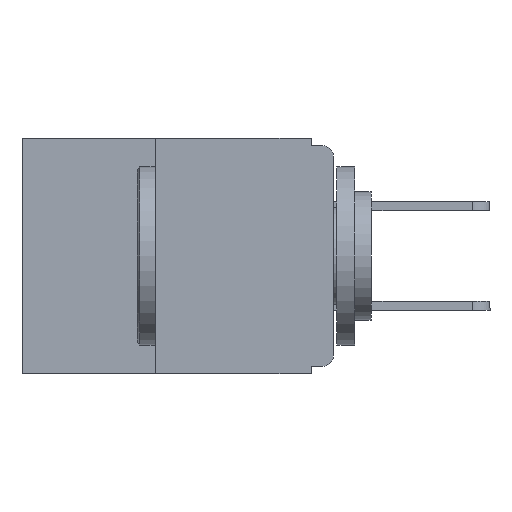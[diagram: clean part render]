
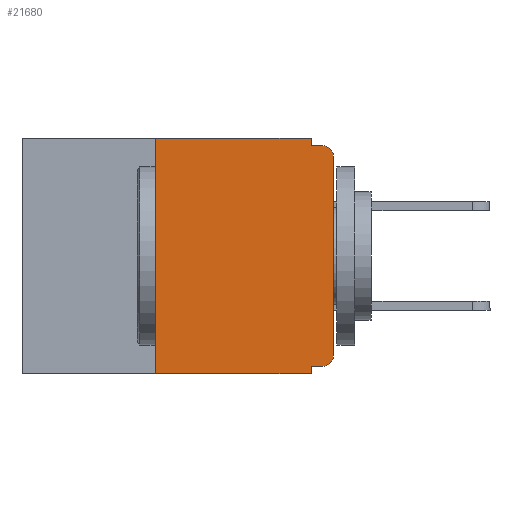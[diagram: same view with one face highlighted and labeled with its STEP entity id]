
A CAD part, left-side view. The second image highlights one B-rep face of the part: STEP entity #21680.
In plain terms, the highlighted planar face has unit normal (-1, 0, 0).
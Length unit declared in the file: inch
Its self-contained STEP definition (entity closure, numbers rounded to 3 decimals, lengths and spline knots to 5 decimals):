
#209 = PLANE ( 'NONE',  #31440 ) ;
#312 = DIRECTION ( 'NONE',  ( 0., 0., -1. ) ) ;
#1443 = AXIS2_PLACEMENT_3D ( 'NONE', #21757, #6638, #24270 ) ;
#2248 = ORIENTED_EDGE ( 'NONE', *, *, #5438, .T. ) ;
#3020 = VERTEX_POINT ( 'NONE', #16339 ) ;
#4085 = VECTOR ( 'NONE', #5358, 39.37008 ) ;
#4108 = DIRECTION ( 'NONE',  ( 0., 0., -1. ) ) ;
#4251 = ORIENTED_EDGE ( 'NONE', *, *, #12909, .F. ) ;
#4727 = CARTESIAN_POINT ( 'NONE',  ( 0., 0.437, -0.33 ) ) ;
#5188 = VECTOR ( 'NONE', #17422, 39.37008 ) ;
#5358 = DIRECTION ( 'NONE',  ( 0., 0., 1. ) ) ;
#5438 = EDGE_CURVE ( 'NONE', #30151, #17853, #26292, .T. ) ;
#6176 = DIRECTION ( 'NONE',  ( 0., 0., -1. ) ) ;
#6638 = DIRECTION ( 'NONE',  ( -1., 0., 0. ) ) ;
#7241 = VECTOR ( 'NONE', #6176, 39.37008 ) ;
#7500 = EDGE_CURVE ( 'NONE', #26751, #17238, #28093, .T. ) ;
#7616 = ORIENTED_EDGE ( 'NONE', *, *, #7500, .F. ) ;
#7727 = ORIENTED_EDGE ( 'NONE', *, *, #22279, .T. ) ;
#7857 = VERTEX_POINT ( 'NONE', #17319 ) ;
#8294 = ORIENTED_EDGE ( 'NONE', *, *, #17800, .F. ) ;
#9288 = VECTOR ( 'NONE', #27717, 39.37008 ) ;
#10606 = ORIENTED_EDGE ( 'NONE', *, *, #11639, .T. ) ;
#10917 = EDGE_LOOP ( 'NONE', ( #7727, #2248, #12436, #4251, #28418, #7616, #10606, #8294, #29253, #27120 ) ) ;
#10956 = EDGE_CURVE ( 'NONE', #32414, #18442, #30687, .T. ) ;
#11639 = EDGE_CURVE ( 'NONE', #26751, #3020, #24506, .T. ) ;
#12216 = EDGE_CURVE ( 'NONE', #32414, #7857, #21367, .T. ) ;
#12436 = ORIENTED_EDGE ( 'NONE', *, *, #16873, .F. ) ;
#12699 = VECTOR ( 'NONE', #4108, 39.37008 ) ;
#12820 = CARTESIAN_POINT ( 'NONE',  ( 0., 0., -0.01 ) ) ;
#12909 = EDGE_CURVE ( 'NONE', #22505, #31209, #32461, .T. ) ;
#13097 = CARTESIAN_POINT ( 'NONE',  ( 0., 0.437, 0. ) ) ;
#14546 = DIRECTION ( 'NONE',  ( 0., 0., -1. ) ) ;
#14616 = DIRECTION ( 'NONE',  ( -1., 0., 0. ) ) ;
#14872 = VECTOR ( 'NONE', #15958, 39.37008 ) ;
#15607 = DIRECTION ( 'NONE',  ( 1., 0., 0. ) ) ;
#15958 = DIRECTION ( 'NONE',  ( 0., 0., 1. ) ) ;
#16339 = CARTESIAN_POINT ( 'NONE',  ( 0., 0.031, -0.33 ) ) ;
#16504 = CARTESIAN_POINT ( 'NONE',  ( 0., 0.015, -0.01 ) ) ;
#16729 = VECTOR ( 'NONE', #28045, 39.37008 ) ;
#16873 = EDGE_CURVE ( 'NONE', #31209, #17853, #28426, .T. ) ;
#17238 = VERTEX_POINT ( 'NONE', #21548 ) ;
#17319 = CARTESIAN_POINT ( 'NONE',  ( 0., 0., -0.305 ) ) ;
#17422 = DIRECTION ( 'NONE',  ( 0., -1., 0. ) ) ;
#17514 = LINE ( 'NONE', #25560, #16729 ) ;
#17570 = VECTOR ( 'NONE', #27178, 39.37008 ) ;
#17800 = EDGE_CURVE ( 'NONE', #18442, #3020, #27243, .T. ) ;
#17853 = VERTEX_POINT ( 'NONE', #16504 ) ;
#18347 = AXIS2_PLACEMENT_3D ( 'NONE', #21064, #14616, #14546 ) ;
#18442 = VERTEX_POINT ( 'NONE', #19417 ) ;
#18773 = CARTESIAN_POINT ( 'NONE',  ( 0., 0.031, -0.33 ) ) ;
#19417 = CARTESIAN_POINT ( 'NONE',  ( 0., 0.031, -0.32 ) ) ;
#20491 = CARTESIAN_POINT ( 'NONE',  ( 0., 0., 0. ) ) ;
#21064 = CARTESIAN_POINT ( 'NONE',  ( 0., 0.015, -0.025 ) ) ;
#21367 = CIRCLE ( 'NONE', #1443, 0.015 ) ;
#21548 = CARTESIAN_POINT ( 'NONE',  ( 0., 0.25, 0. ) ) ;
#21585 = FACE_OUTER_BOUND ( 'NONE', #10917, .T. ) ;
#21680 = ADVANCED_FACE ( 'NONE', ( #21585 ), #209, .F. ) ;
#21757 = CARTESIAN_POINT ( 'NONE',  ( 0., 0.015, -0.305 ) ) ;
#22238 = CARTESIAN_POINT ( 'NONE',  ( 0., 0., -0.32 ) ) ;
#22279 = EDGE_CURVE ( 'NONE', #7857, #30151, #23459, .T. ) ;
#22505 = VERTEX_POINT ( 'NONE', #31569 ) ;
#23459 = LINE ( 'NONE', #20491, #4085 ) ;
#24270 = DIRECTION ( 'NONE',  ( 0., 0., -1. ) ) ;
#24329 = CARTESIAN_POINT ( 'NONE',  ( 0., 0.031, 0. ) ) ;
#24506 = LINE ( 'NONE', #4727, #5188 ) ;
#25560 = CARTESIAN_POINT ( 'NONE',  ( 0., 0.437, 0. ) ) ;
#26292 = CIRCLE ( 'NONE', #18347, 0.015 ) ;
#26751 = VERTEX_POINT ( 'NONE', #30353 ) ;
#27120 = ORIENTED_EDGE ( 'NONE', *, *, #12216, .T. ) ;
#27178 = DIRECTION ( 'NONE',  ( 0., 1., 0. ) ) ;
#27243 = LINE ( 'NONE', #18773, #7241 ) ;
#27459 = EDGE_CURVE ( 'NONE', #17238, #22505, #17514, .T. ) ;
#27717 = DIRECTION ( 'NONE',  ( 0., -1., 0. ) ) ;
#27817 = CARTESIAN_POINT ( 'NONE',  ( 0., 0., -0.025 ) ) ;
#28045 = DIRECTION ( 'NONE',  ( 0., -1., 0. ) ) ;
#28093 = LINE ( 'NONE', #30126, #14872 ) ;
#28418 = ORIENTED_EDGE ( 'NONE', *, *, #27459, .F. ) ;
#28426 = LINE ( 'NONE', #12820, #9288 ) ;
#29253 = ORIENTED_EDGE ( 'NONE', *, *, #10956, .F. ) ;
#30011 = CARTESIAN_POINT ( 'NONE',  ( 0., 0.031, -0.01 ) ) ;
#30126 = CARTESIAN_POINT ( 'NONE',  ( 0., 0.25, -0.33 ) ) ;
#30151 = VERTEX_POINT ( 'NONE', #27817 ) ;
#30219 = CARTESIAN_POINT ( 'NONE',  ( 0., 0.015, -0.32 ) ) ;
#30353 = CARTESIAN_POINT ( 'NONE',  ( 0., 0.25, -0.33 ) ) ;
#30687 = LINE ( 'NONE', #22238, #17570 ) ;
#31209 = VERTEX_POINT ( 'NONE', #30011 ) ;
#31440 = AXIS2_PLACEMENT_3D ( 'NONE', #13097, #15607, #312 ) ;
#31569 = CARTESIAN_POINT ( 'NONE',  ( 0., 0.031, 0. ) ) ;
#32414 = VERTEX_POINT ( 'NONE', #30219 ) ;
#32461 = LINE ( 'NONE', #24329, #12699 ) ;
